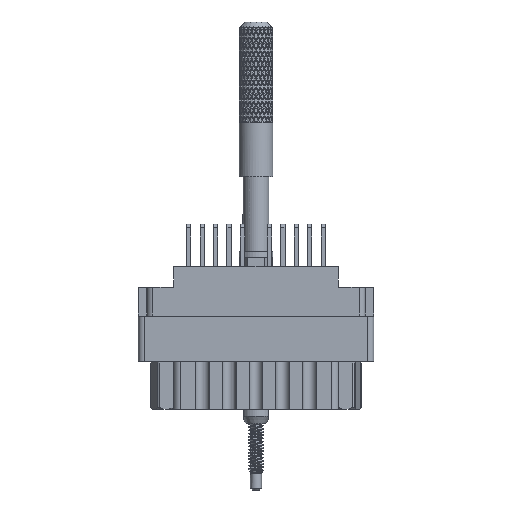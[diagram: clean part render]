
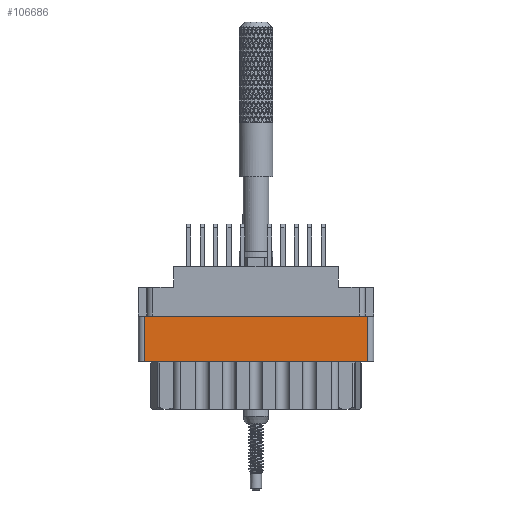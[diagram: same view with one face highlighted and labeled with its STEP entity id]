
A CAD part, front view. The second image highlights one B-rep face of the part: STEP entity #106686.
In plain terms, the highlighted planar face has unit normal (0, -1, 0).
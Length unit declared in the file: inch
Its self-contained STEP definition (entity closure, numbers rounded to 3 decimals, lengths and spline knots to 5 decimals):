
#2107 = CARTESIAN_POINT ( 'NONE',  ( -0.624, -0.343, -0.529 ) ) ;
#2902 = CARTESIAN_POINT ( 'NONE',  ( 0., -0.343, -0.529 ) ) ;
#3278 = EDGE_CURVE ( 'NONE', #97197, #63289, #110517, .T. ) ;
#9061 = VERTEX_POINT ( 'NONE', #140017 ) ;
#15536 = ORIENTED_EDGE ( 'NONE', *, *, #181440, .T. ) ;
#22144 = LINE ( 'NONE', #69902, #178755 ) ;
#24271 = DIRECTION ( 'NONE',  ( -1., 0., 0. ) ) ;
#27115 = EDGE_CURVE ( 'NONE', #9061, #63289, #181320, .T. ) ;
#28492 = CARTESIAN_POINT ( 'NONE',  ( -0.624, -0.343, -0.798 ) ) ;
#29997 = DIRECTION ( 'NONE',  ( 0., 0., 1. ) ) ;
#31317 = CARTESIAN_POINT ( 'NONE',  ( 0.624, -0.343, -0.798 ) ) ;
#38009 = ORIENTED_EDGE ( 'NONE', *, *, #3278, .F. ) ;
#40606 = DIRECTION ( 'NONE',  ( 1., 0., 0. ) ) ;
#48821 = VECTOR ( 'NONE', #29997, 39.37008 ) ;
#49375 = CARTESIAN_POINT ( 'NONE',  ( -0.656, -0.343, -0.798 ) ) ;
#51858 = VERTEX_POINT ( 'NONE', #97108 ) ;
#59472 = PLANE ( 'NONE',  #106426 ) ;
#60258 = VECTOR ( 'NONE', #117582, 39.37008 ) ;
#61432 = DIRECTION ( 'NONE',  ( 0., 0., -1. ) ) ;
#63289 = VERTEX_POINT ( 'NONE', #2107 ) ;
#65291 = VECTOR ( 'NONE', #24271, 39.37008 ) ;
#69902 = CARTESIAN_POINT ( 'NONE',  ( 0., -0.343, -0.277 ) ) ;
#93978 = DIRECTION ( 'NONE',  ( 0., -1., 0. ) ) ;
#97108 = CARTESIAN_POINT ( 'NONE',  ( 0.624, -0.343, -0.277 ) ) ;
#97197 = VERTEX_POINT ( 'NONE', #169093 ) ;
#102657 = ORIENTED_EDGE ( 'NONE', *, *, #171320, .F. ) ;
#106426 = AXIS2_PLACEMENT_3D ( 'NONE', #49375, #93978, #61432 ) ;
#106686 = ADVANCED_FACE ( 'NONE', ( #183288 ), #59472, .T. ) ;
#110517 = LINE ( 'NONE', #2902, #65291 ) ;
#117582 = DIRECTION ( 'NONE',  ( 0., 0., -1. ) ) ;
#140017 = CARTESIAN_POINT ( 'NONE',  ( -0.624, -0.343, -0.277 ) ) ;
#152699 = EDGE_LOOP ( 'NONE', ( #102657, #170270, #38009, #15536 ) ) ;
#169093 = CARTESIAN_POINT ( 'NONE',  ( 0.624, -0.343, -0.529 ) ) ;
#170270 = ORIENTED_EDGE ( 'NONE', *, *, #27115, .T. ) ;
#171320 = EDGE_CURVE ( 'NONE', #9061, #51858, #22144, .T. ) ;
#178755 = VECTOR ( 'NONE', #40606, 39.37008 ) ;
#181320 = LINE ( 'NONE', #28492, #60258 ) ;
#181440 = EDGE_CURVE ( 'NONE', #97197, #51858, #186508, .T. ) ;
#183288 = FACE_OUTER_BOUND ( 'NONE', #152699, .T. ) ;
#186508 = LINE ( 'NONE', #31317, #48821 ) ;
